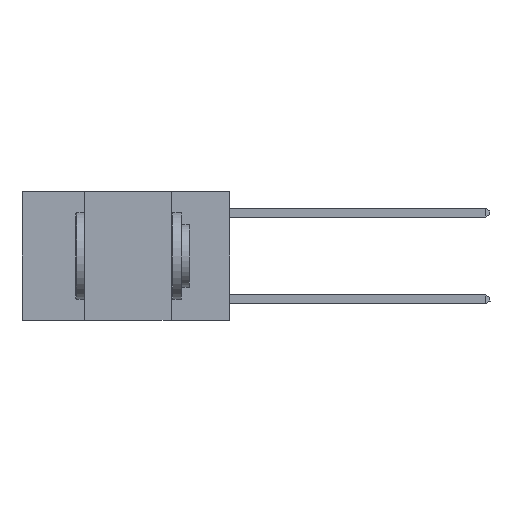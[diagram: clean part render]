
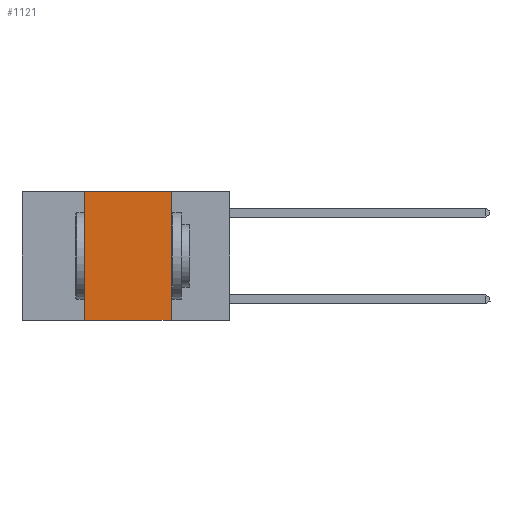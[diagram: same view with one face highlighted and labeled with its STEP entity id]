
A CAD part, left-side view. The second image highlights one B-rep face of the part: STEP entity #1121.
In plain terms, the highlighted planar face has unit normal (-1, 0, 0).
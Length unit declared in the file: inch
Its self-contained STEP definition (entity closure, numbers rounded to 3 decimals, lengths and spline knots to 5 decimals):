
#162 = CARTESIAN_POINT ( 'NONE',  ( 0., 0.42, 0. ) ) ;
#331 = VERTEX_POINT ( 'NONE', #15859 ) ;
#811 = DIRECTION ( 'NONE',  ( 0., -1., 0. ) ) ;
#937 = ORIENTED_EDGE ( 'NONE', *, *, #5045, .F. ) ;
#1005 = DIRECTION ( 'NONE',  ( 1., 0., 0. ) ) ;
#1121 = ADVANCED_FACE ( 'NONE', ( #24219 ), #11702, .F. ) ;
#1793 = CARTESIAN_POINT ( 'NONE',  ( 0., 0.6, 0. ) ) ;
#2010 = DIRECTION ( 'NONE',  ( 0., 0., -1. ) ) ;
#2596 = CARTESIAN_POINT ( 'NONE',  ( 0., 0.17, 0. ) ) ;
#2724 = LINE ( 'NONE', #3872, #3403 ) ;
#3403 = VECTOR ( 'NONE', #8157, 39.37008 ) ;
#3417 = AXIS2_PLACEMENT_3D ( 'NONE', #1793, #1005, #2010 ) ;
#3479 = EDGE_CURVE ( 'NONE', #20826, #331, #2724, .T. ) ;
#3628 = EDGE_CURVE ( 'NONE', #18690, #20826, #15471, .T. ) ;
#3872 = CARTESIAN_POINT ( 'NONE',  ( 0., 0.6, 0. ) ) ;
#4427 = LINE ( 'NONE', #15454, #20289 ) ;
#4711 = EDGE_LOOP ( 'NONE', ( #937, #6598, #17601, #12809 ) ) ;
#5045 = EDGE_CURVE ( 'NONE', #331, #14863, #22051, .T. ) ;
#6598 = ORIENTED_EDGE ( 'NONE', *, *, #3479, .F. ) ;
#6883 = DIRECTION ( 'NONE',  ( 0., 0., -1. ) ) ;
#7490 = CARTESIAN_POINT ( 'NONE',  ( 0., 0.17, -0.37 ) ) ;
#8157 = DIRECTION ( 'NONE',  ( 0., -1., 0. ) ) ;
#11702 = PLANE ( 'NONE',  #3417 ) ;
#12809 = ORIENTED_EDGE ( 'NONE', *, *, #26150, .T. ) ;
#14863 = VERTEX_POINT ( 'NONE', #7490 ) ;
#15454 = CARTESIAN_POINT ( 'NONE',  ( 0., 0.6, -0.37 ) ) ;
#15471 = LINE ( 'NONE', #162, #20243 ) ;
#15859 = CARTESIAN_POINT ( 'NONE',  ( 0., 0.17, 0. ) ) ;
#16691 = VECTOR ( 'NONE', #6883, 39.37008 ) ;
#17324 = CARTESIAN_POINT ( 'NONE',  ( 0., 0.42, -0.37 ) ) ;
#17601 = ORIENTED_EDGE ( 'NONE', *, *, #3628, .F. ) ;
#18690 = VERTEX_POINT ( 'NONE', #17324 ) ;
#18930 = DIRECTION ( 'NONE',  ( 0., 0., 1. ) ) ;
#20243 = VECTOR ( 'NONE', #18930, 39.37008 ) ;
#20289 = VECTOR ( 'NONE', #811, 39.37008 ) ;
#20826 = VERTEX_POINT ( 'NONE', #23987 ) ;
#22051 = LINE ( 'NONE', #2596, #16691 ) ;
#23987 = CARTESIAN_POINT ( 'NONE',  ( 0., 0.42, 0. ) ) ;
#24219 = FACE_OUTER_BOUND ( 'NONE', #4711, .T. ) ;
#26150 = EDGE_CURVE ( 'NONE', #18690, #14863, #4427, .T. ) ;
